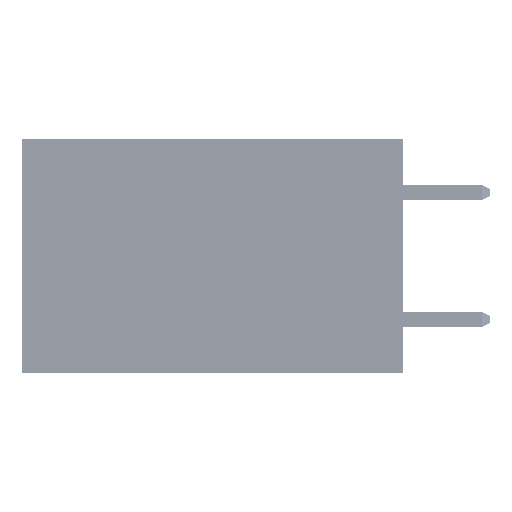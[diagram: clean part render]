
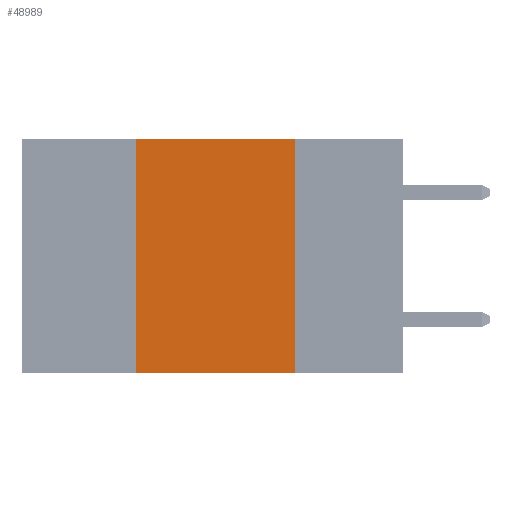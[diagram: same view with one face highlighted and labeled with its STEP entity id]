
A CAD part, left-side view. The second image highlights one B-rep face of the part: STEP entity #48989.
In plain terms, the highlighted planar face has unit normal (-1, 0, 0).
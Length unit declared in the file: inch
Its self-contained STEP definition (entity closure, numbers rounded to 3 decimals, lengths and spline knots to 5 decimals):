
#2884 = DIRECTION ( 'NONE',  ( 0., -1., 0. ) ) ;
#3143 = VERTEX_POINT ( 'NONE', #12321 ) ;
#4034 = DIRECTION ( 'NONE',  ( 0., 0., -1. ) ) ;
#4467 = VECTOR ( 'NONE', #49789, 39.37008 ) ;
#5552 = EDGE_CURVE ( 'NONE', #19274, #26940, #6178, .T. ) ;
#6178 = LINE ( 'NONE', #25075, #28573 ) ;
#8077 = CARTESIAN_POINT ( 'NONE',  ( 0., 0.6, 0. ) ) ;
#9708 = DIRECTION ( 'NONE',  ( 0., 0., -1. ) ) ;
#10984 = ORIENTED_EDGE ( 'NONE', *, *, #5552, .F. ) ;
#12321 = CARTESIAN_POINT ( 'NONE',  ( 0., 0.42, 0. ) ) ;
#13031 = CARTESIAN_POINT ( 'NONE',  ( 0., 0.17, -0.37 ) ) ;
#16694 = ORIENTED_EDGE ( 'NONE', *, *, #33232, .F. ) ;
#19274 = VERTEX_POINT ( 'NONE', #44230 ) ;
#19760 = ORIENTED_EDGE ( 'NONE', *, *, #20588, .T. ) ;
#20588 = EDGE_CURVE ( 'NONE', #38504, #26940, #32867, .T. ) ;
#22050 = LINE ( 'NONE', #36916, #47232 ) ;
#25075 = CARTESIAN_POINT ( 'NONE',  ( 0., 0.17, 0. ) ) ;
#26822 = CARTESIAN_POINT ( 'NONE',  ( 0., 0.42, 0. ) ) ;
#26940 = VERTEX_POINT ( 'NONE', #13031 ) ;
#27467 = PLANE ( 'NONE',  #31822 ) ;
#28573 = VECTOR ( 'NONE', #9708, 39.37008 ) ;
#29039 = ORIENTED_EDGE ( 'NONE', *, *, #32034, .F. ) ;
#31822 = AXIS2_PLACEMENT_3D ( 'NONE', #8077, #34285, #4034 ) ;
#32034 = EDGE_CURVE ( 'NONE', #38504, #3143, #45744, .T. ) ;
#32321 = CARTESIAN_POINT ( 'NONE',  ( 0., 0.42, -0.37 ) ) ;
#32867 = LINE ( 'NONE', #33106, #44152 ) ;
#33106 = CARTESIAN_POINT ( 'NONE',  ( 0., 0.6, -0.37 ) ) ;
#33232 = EDGE_CURVE ( 'NONE', #3143, #19274, #22050, .T. ) ;
#33628 = DIRECTION ( 'NONE',  ( 0., -1., 0. ) ) ;
#34285 = DIRECTION ( 'NONE',  ( 1., 0., 0. ) ) ;
#36392 = EDGE_LOOP ( 'NONE', ( #10984, #16694, #29039, #19760 ) ) ;
#36916 = CARTESIAN_POINT ( 'NONE',  ( 0., 0.6, 0. ) ) ;
#37818 = FACE_OUTER_BOUND ( 'NONE', #36392, .T. ) ;
#38504 = VERTEX_POINT ( 'NONE', #32321 ) ;
#44152 = VECTOR ( 'NONE', #2884, 39.37008 ) ;
#44230 = CARTESIAN_POINT ( 'NONE',  ( 0., 0.17, 0. ) ) ;
#45744 = LINE ( 'NONE', #26822, #4467 ) ;
#47232 = VECTOR ( 'NONE', #33628, 39.37008 ) ;
#48989 = ADVANCED_FACE ( 'NONE', ( #37818 ), #27467, .F. ) ;
#49789 = DIRECTION ( 'NONE',  ( 0., 0., 1. ) ) ;
